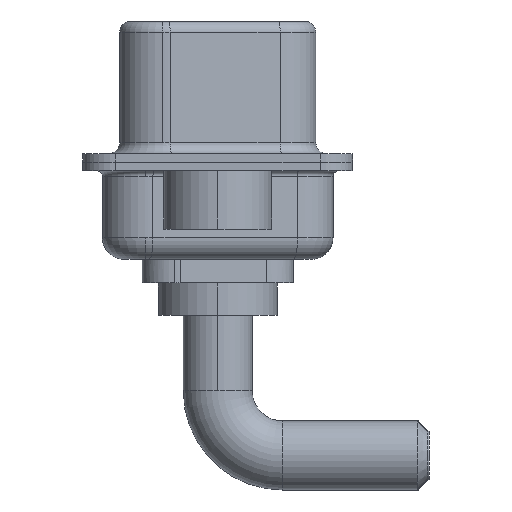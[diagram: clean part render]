
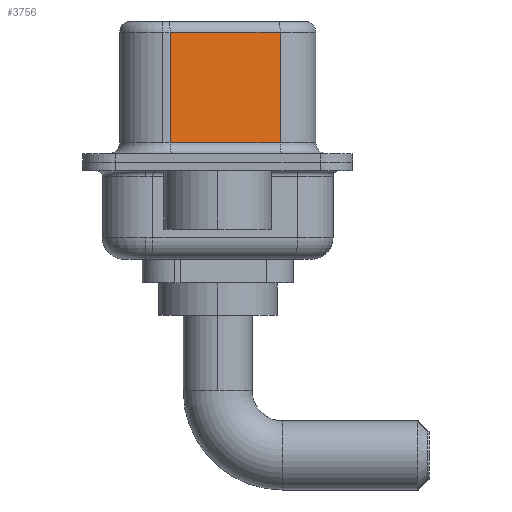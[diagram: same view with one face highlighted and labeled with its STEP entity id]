
A CAD part, left-side view. The second image highlights one B-rep face of the part: STEP entity #3756.
In plain terms, the highlighted planar face has unit normal (-0.985, -0.174, 0).
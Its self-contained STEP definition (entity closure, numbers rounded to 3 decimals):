
#202 = CARTESIAN_POINT ( 'NONE',  ( 3.68, 2.203, 6.02 ) ) ;
#347 = DIRECTION ( 'NONE',  ( 0., 0., -1. ) ) ;
#1275 = DIRECTION ( 'NONE',  ( -0.174, 0.985, 0. ) ) ;
#1856 = CARTESIAN_POINT ( 'NONE',  ( 4.58, -2.897, 0.9 ) ) ;
#2364 = LINE ( 'NONE', #11246, #2717 ) ;
#2496 = CARTESIAN_POINT ( 'NONE',  ( 3.68, 2.203, 6.52 ) ) ;
#2717 = VECTOR ( 'NONE', #1275, 1000. ) ;
#2983 = VERTEX_POINT ( 'NONE', #5599 ) ;
#3470 = VERTEX_POINT ( 'NONE', #4486 ) ;
#3756 = ADVANCED_FACE ( 'NONE', ( #10824 ), #14173, .F. ) ;
#3887 = VECTOR ( 'NONE', #347, 1000. ) ;
#4036 = CARTESIAN_POINT ( 'NONE',  ( 4.58, -2.897, 6.52 ) ) ;
#4188 = DIRECTION ( 'NONE',  ( 0.985, 0.174, 0. ) ) ;
#4324 = VECTOR ( 'NONE', #6237, 1000. ) ;
#4486 = CARTESIAN_POINT ( 'NONE',  ( 4.58, -2.897, 0.9 ) ) ;
#5162 = ORIENTED_EDGE ( 'NONE', *, *, #6370, .T. ) ;
#5258 = VECTOR ( 'NONE', #9054, 1000. ) ;
#5486 = EDGE_CURVE ( 'NONE', #11650, #2983, #7880, .T. ) ;
#5599 = CARTESIAN_POINT ( 'NONE',  ( 3.68, 2.203, 0.9 ) ) ;
#5907 = AXIS2_PLACEMENT_3D ( 'NONE', #4036, #4188, #9726 ) ;
#6161 = CARTESIAN_POINT ( 'NONE',  ( 4.58, -2.897, 6.52 ) ) ;
#6237 = DIRECTION ( 'NONE',  ( 0.174, -0.985, 0. ) ) ;
#6370 = EDGE_CURVE ( 'NONE', #13520, #11650, #2364, .T. ) ;
#7880 = LINE ( 'NONE', #2496, #5258 ) ;
#8347 = LINE ( 'NONE', #6161, #3887 ) ;
#9054 = DIRECTION ( 'NONE',  ( 0., 0., -1. ) ) ;
#9158 = ORIENTED_EDGE ( 'NONE', *, *, #10244, .T. ) ;
#9483 = ORIENTED_EDGE ( 'NONE', *, *, #5486, .T. ) ;
#9726 = DIRECTION ( 'NONE',  ( -0.174, 0.985, 0. ) ) ;
#10244 = EDGE_CURVE ( 'NONE', #2983, #3470, #13796, .T. ) ;
#10659 = CARTESIAN_POINT ( 'NONE',  ( 4.58, -2.897, 6.02 ) ) ;
#10824 = FACE_OUTER_BOUND ( 'NONE', #13565, .T. ) ;
#11246 = CARTESIAN_POINT ( 'NONE',  ( 4.58, -2.897, 6.02 ) ) ;
#11648 = ORIENTED_EDGE ( 'NONE', *, *, #11896, .F. ) ;
#11650 = VERTEX_POINT ( 'NONE', #202 ) ;
#11896 = EDGE_CURVE ( 'NONE', #13520, #3470, #8347, .T. ) ;
#13520 = VERTEX_POINT ( 'NONE', #10659 ) ;
#13565 = EDGE_LOOP ( 'NONE', ( #11648, #5162, #9483, #9158 ) ) ;
#13796 = LINE ( 'NONE', #1856, #4324 ) ;
#14173 = PLANE ( 'NONE',  #5907 ) ;
